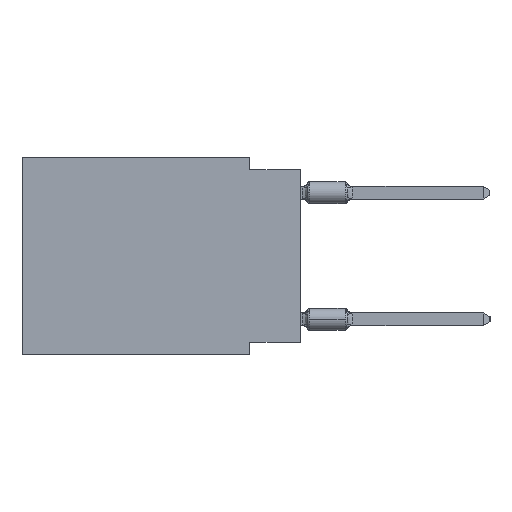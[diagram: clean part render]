
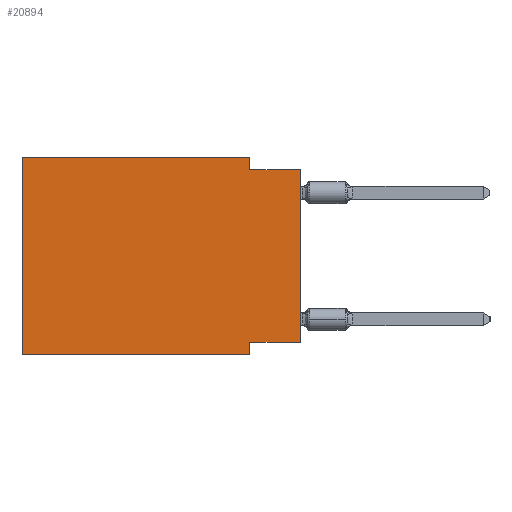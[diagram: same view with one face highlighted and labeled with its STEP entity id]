
A CAD part, left-side view. The second image highlights one B-rep face of the part: STEP entity #20894.
In plain terms, the highlighted planar face has unit normal (-1, 0, 0).
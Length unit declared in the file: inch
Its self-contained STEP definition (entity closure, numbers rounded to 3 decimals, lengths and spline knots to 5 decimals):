
#141 = EDGE_CURVE ( 'NONE', #16277, #30945, #41734, .T. ) ;
#339 = VERTEX_POINT ( 'NONE', #15386 ) ;
#542 = CARTESIAN_POINT ( 'NONE',  ( 0., 0.55, -0.39 ) ) ;
#805 = DIRECTION ( 'NONE',  ( 0., -1., 0. ) ) ;
#1705 = LINE ( 'NONE', #41055, #34274 ) ;
#2118 = ORIENTED_EDGE ( 'NONE', *, *, #33063, .F. ) ;
#2624 = AXIS2_PLACEMENT_3D ( 'NONE', #38487, #30249, #11199 ) ;
#2739 = FACE_OUTER_BOUND ( 'NONE', #16888, .T. ) ;
#3247 = PLANE ( 'NONE',  #2624 ) ;
#6546 = VERTEX_POINT ( 'NONE', #18062 ) ;
#6705 = CARTESIAN_POINT ( 'NONE',  ( 0., 0., 0. ) ) ;
#7239 = LINE ( 'NONE', #542, #38028 ) ;
#7973 = VERTEX_POINT ( 'NONE', #37068 ) ;
#8271 = CARTESIAN_POINT ( 'NONE',  ( 0., 0.55, 0. ) ) ;
#8446 = DIRECTION ( 'NONE',  ( 0., -1., 0. ) ) ;
#8693 = CARTESIAN_POINT ( 'NONE',  ( 0., 0., -0.025 ) ) ;
#9916 = DIRECTION ( 'NONE',  ( 0., 1., 0. ) ) ;
#11199 = DIRECTION ( 'NONE',  ( 0., 0., -1. ) ) ;
#11466 = EDGE_CURVE ( 'NONE', #46405, #339, #16157, .T. ) ;
#12320 = VERTEX_POINT ( 'NONE', #21085 ) ;
#13818 = VECTOR ( 'NONE', #22370, 39.37008 ) ;
#14190 = VECTOR ( 'NONE', #27722, 39.37008 ) ;
#14408 = ORIENTED_EDGE ( 'NONE', *, *, #11466, .F. ) ;
#15386 = CARTESIAN_POINT ( 'NONE',  ( 0., 0., -0.025 ) ) ;
#15500 = EDGE_CURVE ( 'NONE', #12320, #339, #34463, .T. ) ;
#16157 = LINE ( 'NONE', #8693, #36676 ) ;
#16277 = VERTEX_POINT ( 'NONE', #32587 ) ;
#16888 = EDGE_LOOP ( 'NONE', ( #42449, #14408, #19697, #37198, #2118, #44971, #34692, #37591 ) ) ;
#18062 = CARTESIAN_POINT ( 'NONE',  ( 0., 0.1, -0.365 ) ) ;
#19697 = ORIENTED_EDGE ( 'NONE', *, *, #43650, .F. ) ;
#20512 = CARTESIAN_POINT ( 'NONE',  ( 0., 0.1, 0. ) ) ;
#20894 = ADVANCED_FACE ( 'NONE', ( #2739 ), #3247, .F. ) ;
#21085 = CARTESIAN_POINT ( 'NONE',  ( 0., 0., -0.365 ) ) ;
#21820 = EDGE_CURVE ( 'NONE', #7973, #34373, #7239, .T. ) ;
#22370 = DIRECTION ( 'NONE',  ( 0., 0., 1. ) ) ;
#23524 = DIRECTION ( 'NONE',  ( 0., 0., -1. ) ) ;
#27050 = LINE ( 'NONE', #8271, #32000 ) ;
#27722 = DIRECTION ( 'NONE',  ( 0., 0., -1. ) ) ;
#30249 = DIRECTION ( 'NONE',  ( 1., 0., 0. ) ) ;
#30945 = VERTEX_POINT ( 'NONE', #47256 ) ;
#32000 = VECTOR ( 'NONE', #46593, 39.37008 ) ;
#32587 = CARTESIAN_POINT ( 'NONE',  ( 0., 0.55, 0. ) ) ;
#33063 = EDGE_CURVE ( 'NONE', #7973, #16277, #27050, .T. ) ;
#34274 = VECTOR ( 'NONE', #9916, 39.37008 ) ;
#34373 = VERTEX_POINT ( 'NONE', #39918 ) ;
#34378 = VECTOR ( 'NONE', #23524, 39.37008 ) ;
#34463 = LINE ( 'NONE', #6705, #13818 ) ;
#34501 = CARTESIAN_POINT ( 'NONE',  ( 0., 0.55, 0. ) ) ;
#34692 = ORIENTED_EDGE ( 'NONE', *, *, #50372, .F. ) ;
#35352 = EDGE_CURVE ( 'NONE', #12320, #6546, #1705, .T. ) ;
#36676 = VECTOR ( 'NONE', #8446, 39.37008 ) ;
#37068 = CARTESIAN_POINT ( 'NONE',  ( 0., 0.55, -0.39 ) ) ;
#37198 = ORIENTED_EDGE ( 'NONE', *, *, #141, .F. ) ;
#37591 = ORIENTED_EDGE ( 'NONE', *, *, #35352, .F. ) ;
#37869 = DIRECTION ( 'NONE',  ( 0., -1., 0. ) ) ;
#38028 = VECTOR ( 'NONE', #805, 39.37008 ) ;
#38468 = LINE ( 'NONE', #50027, #34378 ) ;
#38487 = CARTESIAN_POINT ( 'NONE',  ( 0., 0.55, 0. ) ) ;
#39918 = CARTESIAN_POINT ( 'NONE',  ( 0., 0.1, -0.39 ) ) ;
#41055 = CARTESIAN_POINT ( 'NONE',  ( 0., 0., -0.365 ) ) ;
#41734 = LINE ( 'NONE', #34501, #49278 ) ;
#42449 = ORIENTED_EDGE ( 'NONE', *, *, #15500, .T. ) ;
#43650 = EDGE_CURVE ( 'NONE', #30945, #46405, #44200, .T. ) ;
#44200 = LINE ( 'NONE', #20512, #14190 ) ;
#44878 = CARTESIAN_POINT ( 'NONE',  ( 0., 0.1, -0.025 ) ) ;
#44971 = ORIENTED_EDGE ( 'NONE', *, *, #21820, .T. ) ;
#46405 = VERTEX_POINT ( 'NONE', #44878 ) ;
#46593 = DIRECTION ( 'NONE',  ( 0., 0., 1. ) ) ;
#47256 = CARTESIAN_POINT ( 'NONE',  ( 0., 0.1, 0. ) ) ;
#49278 = VECTOR ( 'NONE', #37869, 39.37008 ) ;
#50027 = CARTESIAN_POINT ( 'NONE',  ( 0., 0.1, -0.39 ) ) ;
#50372 = EDGE_CURVE ( 'NONE', #6546, #34373, #38468, .T. ) ;
